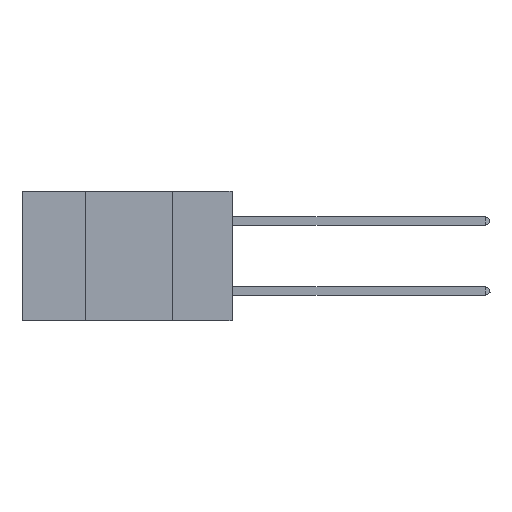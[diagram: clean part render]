
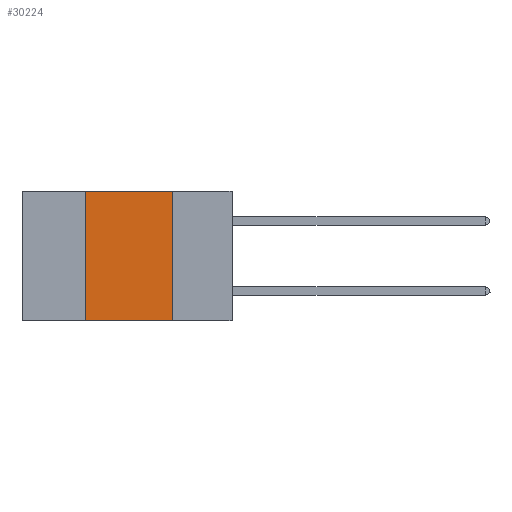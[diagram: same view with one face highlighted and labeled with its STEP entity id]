
A CAD part, left-side view. The second image highlights one B-rep face of the part: STEP entity #30224.
In plain terms, the highlighted planar face has unit normal (-1, 0, 0).
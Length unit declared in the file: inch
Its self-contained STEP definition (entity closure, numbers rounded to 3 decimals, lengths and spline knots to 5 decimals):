
#1328 = PLANE ( 'NONE',  #38826 ) ;
#3646 = CARTESIAN_POINT ( 'NONE',  ( 0., 0.42, 0. ) ) ;
#4516 = VECTOR ( 'NONE', #39275, 39.37008 ) ;
#5145 = EDGE_LOOP ( 'NONE', ( #34353, #28722, #25423, #42866 ) ) ;
#5782 = LINE ( 'NONE', #3646, #4516 ) ;
#8032 = CARTESIAN_POINT ( 'NONE',  ( 0., 0.42, 0. ) ) ;
#8233 = VECTOR ( 'NONE', #30256, 39.37008 ) ;
#8757 = CARTESIAN_POINT ( 'NONE',  ( 0., 0.17, 0. ) ) ;
#12913 = DIRECTION ( 'NONE',  ( 0., 0., -1. ) ) ;
#18112 = VERTEX_POINT ( 'NONE', #20631 ) ;
#20631 = CARTESIAN_POINT ( 'NONE',  ( 0., 0.17, 0. ) ) ;
#21072 = LINE ( 'NONE', #41040, #38048 ) ;
#25423 = ORIENTED_EDGE ( 'NONE', *, *, #43285, .F. ) ;
#26775 = VECTOR ( 'NONE', #32299, 39.37008 ) ;
#27857 = DIRECTION ( 'NONE',  ( 0., -1., 0. ) ) ;
#28584 = CARTESIAN_POINT ( 'NONE',  ( 0., 0.42, -0.37 ) ) ;
#28722 = ORIENTED_EDGE ( 'NONE', *, *, #31576, .F. ) ;
#30224 = ADVANCED_FACE ( 'NONE', ( #43415 ), #1328, .F. ) ;
#30256 = DIRECTION ( 'NONE',  ( 0., 0., -1. ) ) ;
#30598 = EDGE_CURVE ( 'NONE', #31755, #31243, #35717, .T. ) ;
#31243 = VERTEX_POINT ( 'NONE', #35634 ) ;
#31576 = EDGE_CURVE ( 'NONE', #33791, #18112, #21072, .T. ) ;
#31755 = VERTEX_POINT ( 'NONE', #28584 ) ;
#32299 = DIRECTION ( 'NONE',  ( 0., -1., 0. ) ) ;
#33791 = VERTEX_POINT ( 'NONE', #8032 ) ;
#33804 = DIRECTION ( 'NONE',  ( 1., 0., 0. ) ) ;
#34353 = ORIENTED_EDGE ( 'NONE', *, *, #41655, .F. ) ;
#35634 = CARTESIAN_POINT ( 'NONE',  ( 0., 0.17, -0.37 ) ) ;
#35717 = LINE ( 'NONE', #45211, #26775 ) ;
#38048 = VECTOR ( 'NONE', #27857, 39.37008 ) ;
#38826 = AXIS2_PLACEMENT_3D ( 'NONE', #43556, #33804, #12913 ) ;
#39275 = DIRECTION ( 'NONE',  ( 0., 0., 1. ) ) ;
#41040 = CARTESIAN_POINT ( 'NONE',  ( 0., 0.6, 0. ) ) ;
#41655 = EDGE_CURVE ( 'NONE', #18112, #31243, #44954, .T. ) ;
#42866 = ORIENTED_EDGE ( 'NONE', *, *, #30598, .T. ) ;
#43285 = EDGE_CURVE ( 'NONE', #31755, #33791, #5782, .T. ) ;
#43415 = FACE_OUTER_BOUND ( 'NONE', #5145, .T. ) ;
#43556 = CARTESIAN_POINT ( 'NONE',  ( 0., 0.6, 0. ) ) ;
#44954 = LINE ( 'NONE', #8757, #8233 ) ;
#45211 = CARTESIAN_POINT ( 'NONE',  ( 0., 0.6, -0.37 ) ) ;
